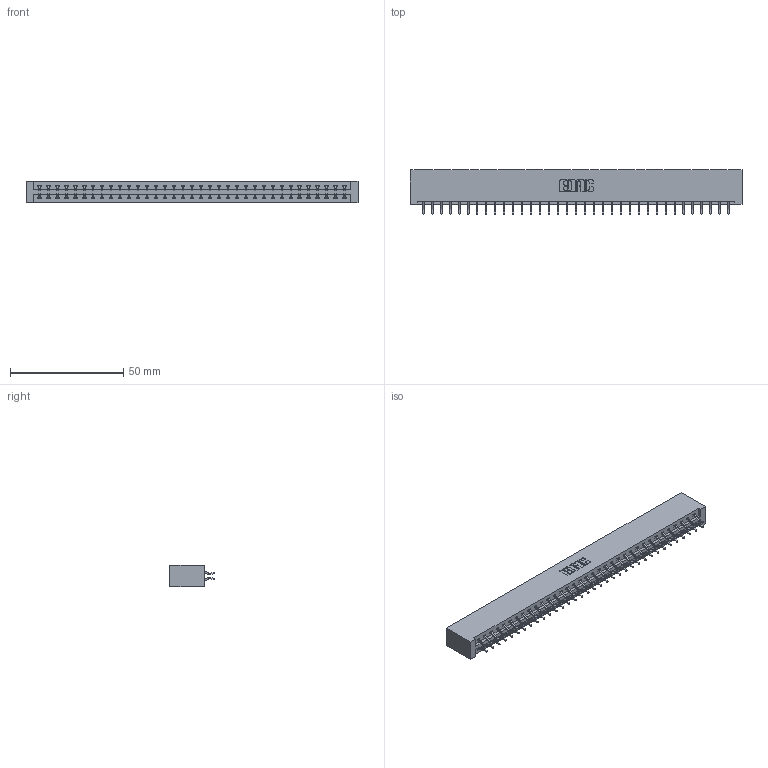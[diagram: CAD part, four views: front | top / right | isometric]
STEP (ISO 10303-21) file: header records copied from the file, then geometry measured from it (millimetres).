
FILE_DESCRIPTION (( 'STEP AP203' ), '1' );
FILE_NAME ('337-070-556-201.STEP', '2018-08-11T12:57:49', ( '' ), ( '' ), 'SwSTEP 2.0', 'SolidWorks 2016', '' );
FILE_SCHEMA (( 'CONFIG_CONTROL_DESIGN' ));
Length unit declared in the file: inch
Products named in the file (3): 337 Part_No Mounting Lugs; 345-292-001_556 Tail; 337-070-556-201
Assembly tree (71 placements, depth 2):
  337-070-556-201
    337 Part_No Mounting Lugs
    345-292-001_556 Tail  x70
Bounding box: 146.56 x 19.57 x 9.4 mm (x, y, z)
Volume: 16110.2 mm3; surface area: 18126.9 mm2
Topology: 71 solids, 71 shells, 4306 faces, 12817 edges, 8450 vertices
Faces by surface type: plane 3006, cylinder 1300
Entity records: 27985 total; most frequent: CARTESIAN_POINT 4734, ORIENTED_EDGE 4658, DIRECTION 4021, EDGE_CURVE 2329, LINE 2201, VECTOR 2201, VERTEX_POINT 1550, AXIS2_PLACEMENT_3D 910
